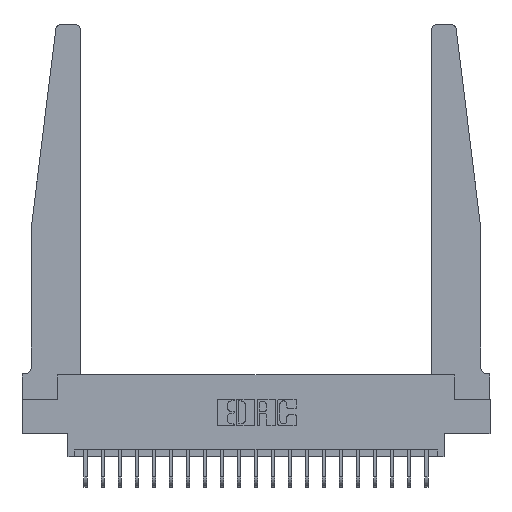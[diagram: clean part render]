
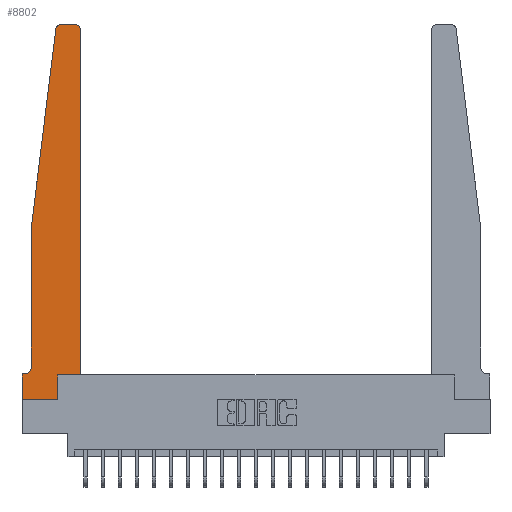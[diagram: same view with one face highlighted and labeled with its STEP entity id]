
A CAD part, top view. The second image highlights one B-rep face of the part: STEP entity #8802.
In plain terms, the highlighted planar face has unit normal (0, 0, 1).
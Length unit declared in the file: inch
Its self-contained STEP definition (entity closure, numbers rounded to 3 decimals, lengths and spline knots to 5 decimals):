
#989 = CARTESIAN_POINT ( 'NONE',  ( 0.395, 2.75, 0.37 ) ) ;
#1281 = EDGE_CURVE ( 'NONE', #8024, #1977, #21466, .T. ) ;
#1378 = CARTESIAN_POINT ( 'NONE',  ( 0., 0., 0.37 ) ) ;
#1486 = CARTESIAN_POINT ( 'NONE',  ( 0.065, 0.1875, 0.37 ) ) ;
#1521 = CARTESIAN_POINT ( 'NONE',  ( 0.015, 0.1875, 0.37 ) ) ;
#1709 = CARTESIAN_POINT ( 'NONE',  ( 0.065, 1.25, 0.37 ) ) ;
#1784 = VERTEX_POINT ( 'NONE', #23480 ) ;
#1977 = VERTEX_POINT ( 'NONE', #13616 ) ;
#2094 = CARTESIAN_POINT ( 'NONE',  ( 0.425, 2.72, 0.37 ) ) ;
#2355 = DIRECTION ( 'NONE',  ( 0., 1., 0. ) ) ;
#2894 = CARTESIAN_POINT ( 'NONE',  ( 0.395, 2.72, 0.37 ) ) ;
#3015 = DIRECTION ( 'NONE',  ( 1., 0., 0. ) ) ;
#3146 = AXIS2_PLACEMENT_3D ( 'NONE', #8403, #6281, #15449 ) ;
#3405 = DIRECTION ( 'NONE',  ( -1., 0., 0. ) ) ;
#4480 = LINE ( 'NONE', #9979, #20788 ) ;
#5046 = VERTEX_POINT ( 'NONE', #2094 ) ;
#5298 = VECTOR ( 'NONE', #18733, 39.37008 ) ;
#5316 = LINE ( 'NONE', #18106, #13054 ) ;
#5333 = DIRECTION ( 'NONE',  ( 0., -1., 0. ) ) ;
#5650 = CARTESIAN_POINT ( 'NONE',  ( 0.2605, 0., 0.37 ) ) ;
#6032 = VECTOR ( 'NONE', #13510, 39.37008 ) ;
#6281 = DIRECTION ( 'NONE',  ( 0., 0., 1. ) ) ;
#7241 = DIRECTION ( 'NONE',  ( 0., 0., 1. ) ) ;
#7854 = ORIENTED_EDGE ( 'NONE', *, *, #8554, .T. ) ;
#8014 = CARTESIAN_POINT ( 'NONE',  ( 0., 0., 0.37 ) ) ;
#8024 = VERTEX_POINT ( 'NONE', #1521 ) ;
#8403 = CARTESIAN_POINT ( 'NONE',  ( 0., 0.1875, 0.37 ) ) ;
#8554 = EDGE_CURVE ( 'NONE', #18628, #8024, #9259, .T. ) ;
#8563 = EDGE_CURVE ( 'NONE', #12376, #23461, #5316, .T. ) ;
#8802 = ADVANCED_FACE ( 'NONE', ( #17254 ), #20966, .T. ) ;
#8909 = CIRCLE ( 'NONE', #13506, 0.03 ) ;
#8919 = ORIENTED_EDGE ( 'NONE', *, *, #17858, .T. ) ;
#9259 = CIRCLE ( 'NONE', #13463, 0.05 ) ;
#9537 = ORIENTED_EDGE ( 'NONE', *, *, #20987, .T. ) ;
#9645 = ORIENTED_EDGE ( 'NONE', *, *, #13516, .T. ) ;
#9772 = LINE ( 'NONE', #13603, #5298 ) ;
#9979 = CARTESIAN_POINT ( 'NONE',  ( 0.425, 0.18, 0.37 ) ) ;
#10101 = DIRECTION ( 'NONE',  ( 0., 1., 0. ) ) ;
#10188 = DIRECTION ( 'NONE',  ( 0., 0., 1. ) ) ;
#10344 = VERTEX_POINT ( 'NONE', #5650 ) ;
#10353 = DIRECTION ( 'NONE',  ( 1., 0., 0. ) ) ;
#10594 = VECTOR ( 'NONE', #12381, 39.37008 ) ;
#11575 = AXIS2_PLACEMENT_3D ( 'NONE', #2894, #10188, #3015 ) ;
#11579 = ORIENTED_EDGE ( 'NONE', *, *, #1281, .T. ) ;
#11706 = VERTEX_POINT ( 'NONE', #18056 ) ;
#12039 = ORIENTED_EDGE ( 'NONE', *, *, #23519, .T. ) ;
#12046 = ORIENTED_EDGE ( 'NONE', *, *, #19897, .T. ) ;
#12376 = VERTEX_POINT ( 'NONE', #989 ) ;
#12381 = DIRECTION ( 'NONE',  ( -1., 0., 0. ) ) ;
#12487 = CARTESIAN_POINT ( 'NONE',  ( 0.015, 0.2375, 0.37 ) ) ;
#12488 = DIRECTION ( 'NONE',  ( 1., 0., 0. ) ) ;
#12858 = VERTEX_POINT ( 'NONE', #22155 ) ;
#13054 = VECTOR ( 'NONE', #21818, 39.37008 ) ;
#13296 = EDGE_CURVE ( 'NONE', #12858, #10344, #23038, .T. ) ;
#13366 = CARTESIAN_POINT ( 'NONE',  ( 0.2605, 0.18, 0.37 ) ) ;
#13463 = AXIS2_PLACEMENT_3D ( 'NONE', #12487, #19783, #3405 ) ;
#13506 = AXIS2_PLACEMENT_3D ( 'NONE', #21583, #7241, #12488 ) ;
#13510 = DIRECTION ( 'NONE',  ( 1., 0., 0. ) ) ;
#13516 = EDGE_CURVE ( 'NONE', #1977, #12858, #21716, .T. ) ;
#13603 = CARTESIAN_POINT ( 'NONE',  ( 0.065, 1.25, 0.37 ) ) ;
#13616 = CARTESIAN_POINT ( 'NONE',  ( 0., 0.1875, 0.37 ) ) ;
#13940 = ORIENTED_EDGE ( 'NONE', *, *, #14966, .T. ) ;
#14401 = CARTESIAN_POINT ( 'NONE',  ( 0.425, 0.18, 0.37 ) ) ;
#14681 = LINE ( 'NONE', #14793, #23044 ) ;
#14793 = CARTESIAN_POINT ( 'NONE',  ( 0.2605, 0.18, 0.37 ) ) ;
#14966 = EDGE_CURVE ( 'NONE', #1784, #11706, #9772, .T. ) ;
#15449 = DIRECTION ( 'NONE',  ( 1., 0., 0. ) ) ;
#15559 = ORIENTED_EDGE ( 'NONE', *, *, #13296, .T. ) ;
#15941 = CARTESIAN_POINT ( 'NONE',  ( 0.27653, 2.75, 0.37 ) ) ;
#16071 = LINE ( 'NONE', #14401, #23482 ) ;
#17034 = VECTOR ( 'NONE', #21574, 39.37008 ) ;
#17186 = VECTOR ( 'NONE', #5333, 39.37008 ) ;
#17254 = FACE_OUTER_BOUND ( 'NONE', #18402, .T. ) ;
#17275 = EDGE_CURVE ( 'NONE', #5046, #12376, #21486, .T. ) ;
#17569 = CARTESIAN_POINT ( 'NONE',  ( 0.425, 0.18, 0.37 ) ) ;
#17665 = VERTEX_POINT ( 'NONE', #17569 ) ;
#17858 = EDGE_CURVE ( 'NONE', #10344, #21767, #14681, .T. ) ;
#17960 = CARTESIAN_POINT ( 'NONE',  ( 0.065, 0.2375, 0.37 ) ) ;
#17981 = LINE ( 'NONE', #1709, #17034 ) ;
#18056 = CARTESIAN_POINT ( 'NONE',  ( 0.065, 1.25, 0.37 ) ) ;
#18106 = CARTESIAN_POINT ( 'NONE',  ( 0.25, 2.75, 0.37 ) ) ;
#18136 = ORIENTED_EDGE ( 'NONE', *, *, #17275, .T. ) ;
#18236 = EDGE_CURVE ( 'NONE', #23461, #1784, #8909, .T. ) ;
#18402 = EDGE_LOOP ( 'NONE', ( #23050, #19923, #13940, #12039, #7854, #11579, #9645, #15559, #8919, #12046, #9537, #18136 ) ) ;
#18628 = VERTEX_POINT ( 'NONE', #17960 ) ;
#18733 = DIRECTION ( 'NONE',  ( -0.122, -0.992, 0. ) ) ;
#19783 = DIRECTION ( 'NONE',  ( 0., 0., -1. ) ) ;
#19897 = EDGE_CURVE ( 'NONE', #21767, #17665, #16071, .T. ) ;
#19923 = ORIENTED_EDGE ( 'NONE', *, *, #18236, .T. ) ;
#20788 = VECTOR ( 'NONE', #10101, 39.37008 ) ;
#20966 = PLANE ( 'NONE',  #3146 ) ;
#20987 = EDGE_CURVE ( 'NONE', #17665, #5046, #4480, .T. ) ;
#21466 = LINE ( 'NONE', #1486, #10594 ) ;
#21486 = CIRCLE ( 'NONE', #11575, 0.03 ) ;
#21574 = DIRECTION ( 'NONE',  ( 0., -1., 0. ) ) ;
#21583 = CARTESIAN_POINT ( 'NONE',  ( 0.27653, 2.72, 0.37 ) ) ;
#21716 = LINE ( 'NONE', #1378, #17186 ) ;
#21767 = VERTEX_POINT ( 'NONE', #13366 ) ;
#21818 = DIRECTION ( 'NONE',  ( -1., 0., 0. ) ) ;
#22155 = CARTESIAN_POINT ( 'NONE',  ( 0., 0., 0.37 ) ) ;
#23038 = LINE ( 'NONE', #8014, #6032 ) ;
#23044 = VECTOR ( 'NONE', #2355, 39.37008 ) ;
#23050 = ORIENTED_EDGE ( 'NONE', *, *, #8563, .T. ) ;
#23461 = VERTEX_POINT ( 'NONE', #15941 ) ;
#23480 = CARTESIAN_POINT ( 'NONE',  ( 0.24675, 2.72367, 0.37 ) ) ;
#23482 = VECTOR ( 'NONE', #10353, 39.37008 ) ;
#23519 = EDGE_CURVE ( 'NONE', #11706, #18628, #17981, .T. ) ;
